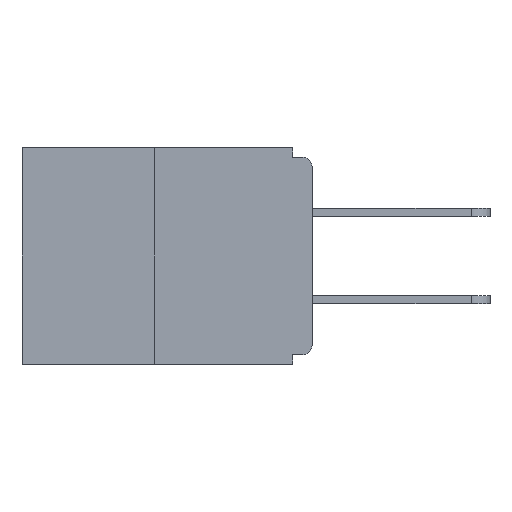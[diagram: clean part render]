
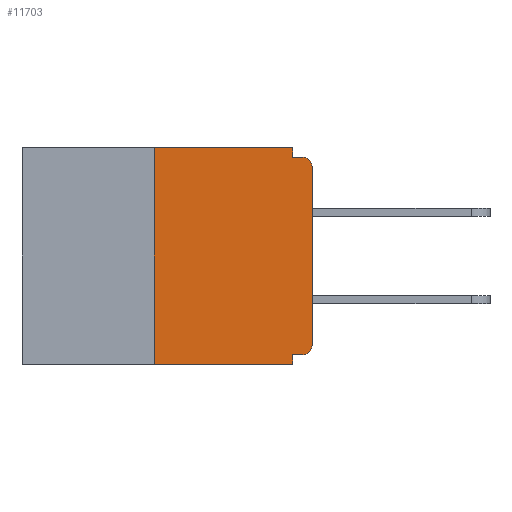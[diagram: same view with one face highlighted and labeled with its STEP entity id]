
A CAD part, left-side view. The second image highlights one B-rep face of the part: STEP entity #11703.
In plain terms, the highlighted planar face has unit normal (-1, 0, 0).
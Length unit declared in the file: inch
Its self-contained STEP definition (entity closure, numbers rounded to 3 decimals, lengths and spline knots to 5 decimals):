
#54 = CARTESIAN_POINT ( 'NONE',  ( 0., 0.25, 0. ) ) ;
#943 = CARTESIAN_POINT ( 'NONE',  ( 0., 0.015, -0.03 ) ) ;
#962 = DIRECTION ( 'NONE',  ( 1., 0., 0. ) ) ;
#1227 = ORIENTED_EDGE ( 'NONE', *, *, #12913, .T. ) ;
#1232 = VECTOR ( 'NONE', #5528, 39.37008 ) ;
#1298 = AXIS2_PLACEMENT_3D ( 'NONE', #2742, #21525, #21420 ) ;
#1425 = CARTESIAN_POINT ( 'NONE',  ( 0., 0.015, -0.328 ) ) ;
#1427 = VERTEX_POINT ( 'NONE', #26797 ) ;
#1431 = DIRECTION ( 'NONE',  ( 0., -1., 0. ) ) ;
#1676 = EDGE_CURVE ( 'NONE', #15503, #16372, #1878, .T. ) ;
#1802 = ORIENTED_EDGE ( 'NONE', *, *, #20110, .F. ) ;
#1878 = LINE ( 'NONE', #8600, #1232 ) ;
#2742 = CARTESIAN_POINT ( 'NONE',  ( 0., 0.015, -0.313 ) ) ;
#3465 = VECTOR ( 'NONE', #9915, 39.37008 ) ;
#3628 = CARTESIAN_POINT ( 'NONE',  ( 0., 0., -0.328 ) ) ;
#4140 = CARTESIAN_POINT ( 'NONE',  ( 0., 0.031, -0.015 ) ) ;
#4724 = VERTEX_POINT ( 'NONE', #18264 ) ;
#4920 = LINE ( 'NONE', #3628, #6560 ) ;
#5172 = FACE_OUTER_BOUND ( 'NONE', #6112, .T. ) ;
#5207 = EDGE_CURVE ( 'NONE', #21805, #15503, #24942, .T. ) ;
#5214 = CARTESIAN_POINT ( 'NONE',  ( 0., 0.015, -0.015 ) ) ;
#5313 = CARTESIAN_POINT ( 'NONE',  ( 0., 0.25, 0. ) ) ;
#5528 = DIRECTION ( 'NONE',  ( 0., 0., 1. ) ) ;
#5602 = CIRCLE ( 'NONE', #17393, 0.015 ) ;
#5755 = DIRECTION ( 'NONE',  ( 0., 0., -1. ) ) ;
#5978 = CARTESIAN_POINT ( 'NONE',  ( 0., 0., -0.03 ) ) ;
#6112 = EDGE_LOOP ( 'NONE', ( #7793, #16222, #1227, #21023, #25925, #24273, #25191, #25275, #1802, #13992 ) ) ;
#6560 = VECTOR ( 'NONE', #10002, 39.37008 ) ;
#7196 = LINE ( 'NONE', #5313, #11496 ) ;
#7793 = ORIENTED_EDGE ( 'NONE', *, *, #18750, .F. ) ;
#8192 = VECTOR ( 'NONE', #5755, 39.37008 ) ;
#8448 = VECTOR ( 'NONE', #25284, 39.37008 ) ;
#8600 = CARTESIAN_POINT ( 'NONE',  ( 0., 0., 0. ) ) ;
#9166 = AXIS2_PLACEMENT_3D ( 'NONE', #26799, #962, #15740 ) ;
#9915 = DIRECTION ( 'NONE',  ( 0., -1., 0. ) ) ;
#10002 = DIRECTION ( 'NONE',  ( 0., 1., 0. ) ) ;
#11151 = LINE ( 'NONE', #14437, #8192 ) ;
#11496 = VECTOR ( 'NONE', #17890, 39.37008 ) ;
#11703 = ADVANCED_FACE ( 'NONE', ( #5172 ), #11935, .F. ) ;
#11738 = DIRECTION ( 'NONE',  ( -1., 0., 0. ) ) ;
#11935 = PLANE ( 'NONE',  #9166 ) ;
#12215 = CARTESIAN_POINT ( 'NONE',  ( 0., 0.46, -0.343 ) ) ;
#12913 = EDGE_CURVE ( 'NONE', #4724, #16037, #23701, .T. ) ;
#13513 = VERTEX_POINT ( 'NONE', #54 ) ;
#13992 = ORIENTED_EDGE ( 'NONE', *, *, #19397, .F. ) ;
#14094 = CARTESIAN_POINT ( 'NONE',  ( 0., 0., -0.015 ) ) ;
#14265 = CARTESIAN_POINT ( 'NONE',  ( 0., 0.031, 0. ) ) ;
#14437 = CARTESIAN_POINT ( 'NONE',  ( 0., 0.031, -0.343 ) ) ;
#15493 = EDGE_CURVE ( 'NONE', #16372, #26000, #5602, .T. ) ;
#15503 = VERTEX_POINT ( 'NONE', #22010 ) ;
#15740 = DIRECTION ( 'NONE',  ( 0., 0., -1. ) ) ;
#15893 = DIRECTION ( 'NONE',  ( 0., 0., -1. ) ) ;
#16037 = VERTEX_POINT ( 'NONE', #25052 ) ;
#16099 = LINE ( 'NONE', #14265, #25795 ) ;
#16113 = EDGE_CURVE ( 'NONE', #21805, #23079, #4920, .T. ) ;
#16222 = ORIENTED_EDGE ( 'NONE', *, *, #17206, .F. ) ;
#16372 = VERTEX_POINT ( 'NONE', #5978 ) ;
#17206 = EDGE_CURVE ( 'NONE', #4724, #13513, #7196, .T. ) ;
#17393 = AXIS2_PLACEMENT_3D ( 'NONE', #943, #11738, #15893 ) ;
#17890 = DIRECTION ( 'NONE',  ( 0., 0., 1. ) ) ;
#18264 = CARTESIAN_POINT ( 'NONE',  ( 0., 0.25, -0.343 ) ) ;
#18750 = EDGE_CURVE ( 'NONE', #13513, #1427, #19025, .T. ) ;
#18875 = CARTESIAN_POINT ( 'NONE',  ( 0., 0.031, -0.328 ) ) ;
#19025 = LINE ( 'NONE', #23196, #8448 ) ;
#19397 = EDGE_CURVE ( 'NONE', #1427, #25665, #16099, .T. ) ;
#20054 = VECTOR ( 'NONE', #1431, 39.37008 ) ;
#20110 = EDGE_CURVE ( 'NONE', #25665, #26000, #25746, .T. ) ;
#21023 = ORIENTED_EDGE ( 'NONE', *, *, #26124, .F. ) ;
#21420 = DIRECTION ( 'NONE',  ( 0., 0., -1. ) ) ;
#21525 = DIRECTION ( 'NONE',  ( -1., 0., 0. ) ) ;
#21805 = VERTEX_POINT ( 'NONE', #1425 ) ;
#22010 = CARTESIAN_POINT ( 'NONE',  ( 0., 0., -0.313 ) ) ;
#22985 = DIRECTION ( 'NONE',  ( 0., 0., -1. ) ) ;
#23079 = VERTEX_POINT ( 'NONE', #18875 ) ;
#23196 = CARTESIAN_POINT ( 'NONE',  ( 0., 0.46, 0. ) ) ;
#23701 = LINE ( 'NONE', #12215, #3465 ) ;
#24273 = ORIENTED_EDGE ( 'NONE', *, *, #5207, .T. ) ;
#24942 = CIRCLE ( 'NONE', #1298, 0.015 ) ;
#25052 = CARTESIAN_POINT ( 'NONE',  ( 0., 0.031, -0.343 ) ) ;
#25191 = ORIENTED_EDGE ( 'NONE', *, *, #1676, .T. ) ;
#25275 = ORIENTED_EDGE ( 'NONE', *, *, #15493, .T. ) ;
#25284 = DIRECTION ( 'NONE',  ( 0., -1., 0. ) ) ;
#25665 = VERTEX_POINT ( 'NONE', #4140 ) ;
#25746 = LINE ( 'NONE', #14094, #20054 ) ;
#25795 = VECTOR ( 'NONE', #22985, 39.37008 ) ;
#25925 = ORIENTED_EDGE ( 'NONE', *, *, #16113, .F. ) ;
#26000 = VERTEX_POINT ( 'NONE', #5214 ) ;
#26124 = EDGE_CURVE ( 'NONE', #23079, #16037, #11151, .T. ) ;
#26797 = CARTESIAN_POINT ( 'NONE',  ( 0., 0.031, 0. ) ) ;
#26799 = CARTESIAN_POINT ( 'NONE',  ( 0., 0.46, 0. ) ) ;
